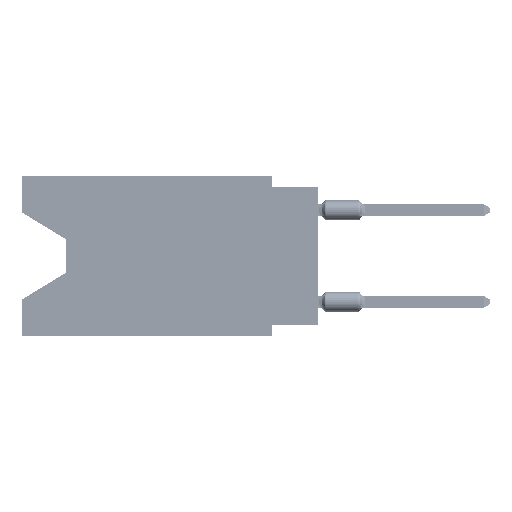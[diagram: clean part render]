
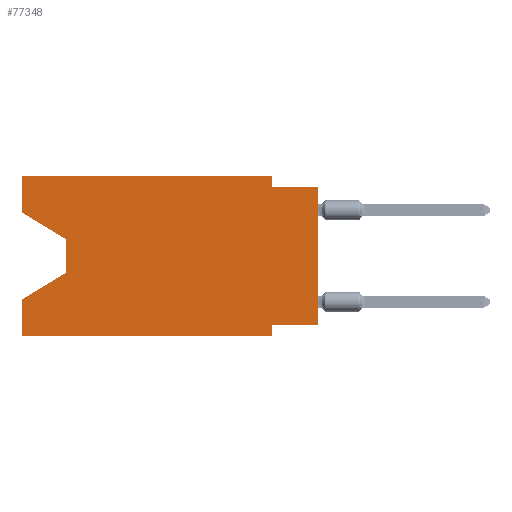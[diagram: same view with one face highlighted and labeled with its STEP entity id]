
A CAD part, left-side view. The second image highlights one B-rep face of the part: STEP entity #77348.
In plain terms, the highlighted planar face has unit normal (-1, 0, 0).
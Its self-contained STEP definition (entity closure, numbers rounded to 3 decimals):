
#469 = LINE ( 'NONE', #70470, #81706 ) ;
#3417 = VECTOR ( 'NONE', #31204, 1000. ) ;
#3918 = CARTESIAN_POINT ( 'NONE',  ( 0., 16.383, 0. ) ) ;
#5031 = DIRECTION ( 'NONE',  ( 0., 0., -1. ) ) ;
#5385 = EDGE_CURVE ( 'NONE', #91303, #79852, #469, .T. ) ;
#5541 = DIRECTION ( 'NONE',  ( 1., 0., 0. ) ) ;
#6938 = LINE ( 'NONE', #30918, #97006 ) ;
#8077 = LINE ( 'NONE', #24249, #66772 ) ;
#8396 = LINE ( 'NONE', #96089, #92620 ) ;
#10167 = CARTESIAN_POINT ( 'NONE',  ( 0., 16.383, -6.852 ) ) ;
#12053 = VECTOR ( 'NONE', #43666, 1000. ) ;
#12217 = CARTESIAN_POINT ( 'NONE',  ( 0., 2.54, -8.255 ) ) ;
#12598 = DIRECTION ( 'NONE',  ( 0., 0., -1. ) ) ;
#12604 = LINE ( 'NONE', #53828, #13363 ) ;
#13363 = VECTOR ( 'NONE', #37117, 1000. ) ;
#13618 = EDGE_CURVE ( 'NONE', #46526, #82527, #8077, .T. ) ;
#14050 = ORIENTED_EDGE ( 'NONE', *, *, #33244, .T. ) ;
#15074 = CARTESIAN_POINT ( 'NONE',  ( 0., 0., -0.635 ) ) ;
#15234 = ORIENTED_EDGE ( 'NONE', *, *, #83748, .T. ) ;
#15269 = EDGE_CURVE ( 'NONE', #102278, #82527, #6938, .T. ) ;
#18518 = ORIENTED_EDGE ( 'NONE', *, *, #15269, .F. ) ;
#18579 = CARTESIAN_POINT ( 'NONE',  ( 0., 16.383, 0. ) ) ;
#21731 = VERTEX_POINT ( 'NONE', #43444 ) ;
#23785 = DIRECTION ( 'NONE',  ( 0., 1., 0. ) ) ;
#24249 = CARTESIAN_POINT ( 'NONE',  ( 0., 13.97, -5.385 ) ) ;
#25522 = VERTEX_POINT ( 'NONE', #18579 ) ;
#26969 = CARTESIAN_POINT ( 'NONE',  ( 0., 0., -8.255 ) ) ;
#30207 = LINE ( 'NONE', #15074, #71964 ) ;
#30918 = CARTESIAN_POINT ( 'NONE',  ( 0., 16.383, 0. ) ) ;
#31204 = DIRECTION ( 'NONE',  ( 0., 0., 1. ) ) ;
#31728 = CARTESIAN_POINT ( 'NONE',  ( 0., 2.54, -8.89 ) ) ;
#33244 = EDGE_CURVE ( 'NONE', #102278, #66309, #49456, .T. ) ;
#33356 = LINE ( 'NONE', #81416, #73720 ) ;
#35563 = VECTOR ( 'NONE', #23785, 1000. ) ;
#36615 = EDGE_CURVE ( 'NONE', #94051, #46176, #8396, .T. ) ;
#37028 = ORIENTED_EDGE ( 'NONE', *, *, #67429, .T. ) ;
#37117 = DIRECTION ( 'NONE',  ( 0., 0., -1. ) ) ;
#37877 = FACE_OUTER_BOUND ( 'NONE', #67607, .T. ) ;
#41402 = ORIENTED_EDGE ( 'NONE', *, *, #13618, .T. ) ;
#43444 = CARTESIAN_POINT ( 'NONE',  ( 0., 0., -0.635 ) ) ;
#43666 = DIRECTION ( 'NONE',  ( 0., -1., 0. ) ) ;
#44044 = EDGE_CURVE ( 'NONE', #25522, #91303, #73938, .T. ) ;
#45339 = DIRECTION ( 'NONE',  ( 0., -1., 0. ) ) ;
#45841 = ORIENTED_EDGE ( 'NONE', *, *, #68058, .F. ) ;
#46176 = VERTEX_POINT ( 'NONE', #52047 ) ;
#46526 = VERTEX_POINT ( 'NONE', #64534 ) ;
#47442 = DIRECTION ( 'NONE',  ( 0., 0., -1. ) ) ;
#47967 = DIRECTION ( 'NONE',  ( 0., 0., 1. ) ) ;
#49456 = LINE ( 'NONE', #90707, #12053 ) ;
#50385 = ORIENTED_EDGE ( 'NONE', *, *, #97442, .F. ) ;
#52047 = CARTESIAN_POINT ( 'NONE',  ( 0., 13.97, -3.505 ) ) ;
#53828 = CARTESIAN_POINT ( 'NONE',  ( 0., 2.54, -8.89 ) ) ;
#54943 = DIRECTION ( 'NONE',  ( 0., 0., 1. ) ) ;
#57258 = CARTESIAN_POINT ( 'NONE',  ( 0., 16.383, -2.038 ) ) ;
#57414 = ORIENTED_EDGE ( 'NONE', *, *, #44044, .F. ) ;
#57630 = DIRECTION ( 'NONE',  ( 0., 0.855, -0.519 ) ) ;
#62182 = CARTESIAN_POINT ( 'NONE',  ( 0., 2.54, 0. ) ) ;
#64534 = CARTESIAN_POINT ( 'NONE',  ( 0., 13.97, -5.385 ) ) ;
#66309 = VERTEX_POINT ( 'NONE', #31728 ) ;
#66772 = VECTOR ( 'NONE', #57630, 1000. ) ;
#67429 = EDGE_CURVE ( 'NONE', #46176, #46526, #68995, .T. ) ;
#67607 = EDGE_LOOP ( 'NONE', ( #97051, #37028, #41402, #18518, #14050, #50385, #94602, #15234, #45841, #80784, #57414, #70622 ) ) ;
#67693 = PLANE ( 'NONE',  #93120 ) ;
#68058 = EDGE_CURVE ( 'NONE', #79852, #21731, #30207, .T. ) ;
#68110 = CARTESIAN_POINT ( 'NONE',  ( 0., 16.383, -8.89 ) ) ;
#68995 = LINE ( 'NONE', #76312, #86871 ) ;
#70289 = LINE ( 'NONE', #79151, #35563 ) ;
#70470 = CARTESIAN_POINT ( 'NONE',  ( 0., 2.54, 0. ) ) ;
#70622 = ORIENTED_EDGE ( 'NONE', *, *, #102948, .F. ) ;
#71438 = LINE ( 'NONE', #79274, #3417 ) ;
#71964 = VECTOR ( 'NONE', #45339, 1000. ) ;
#73720 = VECTOR ( 'NONE', #47967, 1000. ) ;
#73938 = LINE ( 'NONE', #3918, #84501 ) ;
#75528 = CARTESIAN_POINT ( 'NONE',  ( 0., 16.383, 0. ) ) ;
#76068 = CARTESIAN_POINT ( 'NONE',  ( 0., 2.54, -0.635 ) ) ;
#76312 = CARTESIAN_POINT ( 'NONE',  ( 0., 13.97, -3.505 ) ) ;
#77348 = ADVANCED_FACE ( 'NONE', ( #37877 ), #67693, .F. ) ;
#79151 = CARTESIAN_POINT ( 'NONE',  ( 0., 0., -8.255 ) ) ;
#79274 = CARTESIAN_POINT ( 'NONE',  ( 0., 0., 0. ) ) ;
#79852 = VERTEX_POINT ( 'NONE', #76068 ) ;
#80784 = ORIENTED_EDGE ( 'NONE', *, *, #5385, .F. ) ;
#80969 = DIRECTION ( 'NONE',  ( 0., -0.855, -0.519 ) ) ;
#81416 = CARTESIAN_POINT ( 'NONE',  ( 0., 16.383, 0. ) ) ;
#81706 = VECTOR ( 'NONE', #47442, 1000. ) ;
#82527 = VERTEX_POINT ( 'NONE', #10167 ) ;
#83748 = EDGE_CURVE ( 'NONE', #88967, #21731, #71438, .T. ) ;
#83816 = DIRECTION ( 'NONE',  ( 0., -1., 0. ) ) ;
#84501 = VECTOR ( 'NONE', #83816, 1000. ) ;
#86684 = EDGE_CURVE ( 'NONE', #88967, #97165, #70289, .T. ) ;
#86871 = VECTOR ( 'NONE', #12598, 1000. ) ;
#88967 = VERTEX_POINT ( 'NONE', #26969 ) ;
#90707 = CARTESIAN_POINT ( 'NONE',  ( 0., 16.383, -8.89 ) ) ;
#91303 = VERTEX_POINT ( 'NONE', #62182 ) ;
#92620 = VECTOR ( 'NONE', #80969, 1000. ) ;
#93120 = AXIS2_PLACEMENT_3D ( 'NONE', #75528, #5541, #5031 ) ;
#94051 = VERTEX_POINT ( 'NONE', #57258 ) ;
#94602 = ORIENTED_EDGE ( 'NONE', *, *, #86684, .F. ) ;
#96089 = CARTESIAN_POINT ( 'NONE',  ( 0., 16.383, -2.038 ) ) ;
#97006 = VECTOR ( 'NONE', #54943, 1000. ) ;
#97051 = ORIENTED_EDGE ( 'NONE', *, *, #36615, .T. ) ;
#97165 = VERTEX_POINT ( 'NONE', #12217 ) ;
#97442 = EDGE_CURVE ( 'NONE', #97165, #66309, #12604, .T. ) ;
#102278 = VERTEX_POINT ( 'NONE', #68110 ) ;
#102948 = EDGE_CURVE ( 'NONE', #94051, #25522, #33356, .T. ) ;
